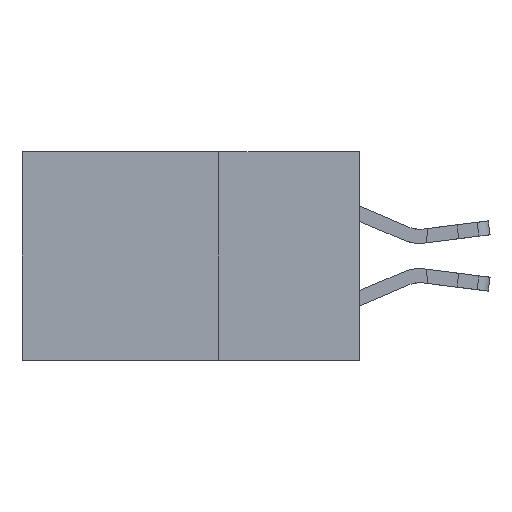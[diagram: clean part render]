
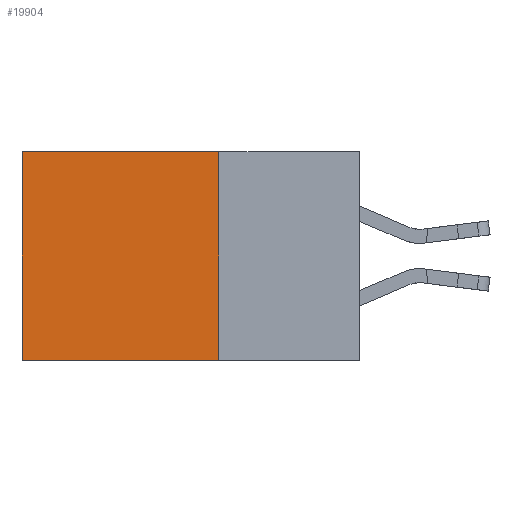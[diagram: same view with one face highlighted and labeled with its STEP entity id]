
A CAD part, left-side view. The second image highlights one B-rep face of the part: STEP entity #19904.
In plain terms, the highlighted planar face has unit normal (-1, 0, 0).
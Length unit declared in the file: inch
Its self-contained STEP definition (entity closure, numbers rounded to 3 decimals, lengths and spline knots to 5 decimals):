
#513 = EDGE_CURVE ( 'NONE', #1936, #17469, #19336, .T. ) ;
#823 = CARTESIAN_POINT ( 'NONE',  ( 0.2875, 0.25, 0. ) ) ;
#1936 = VERTEX_POINT ( 'NONE', #20392 ) ;
#2224 = CARTESIAN_POINT ( 'NONE',  ( 0.2875, 0.6, 0. ) ) ;
#2242 = EDGE_LOOP ( 'NONE', ( #12821, #14230, #16494, #14750 ) ) ;
#2592 = CARTESIAN_POINT ( 'NONE',  ( 0.2875, 0.25, 0. ) ) ;
#2720 = DIRECTION ( 'NONE',  ( 1., 0., 0. ) ) ;
#3605 = CARTESIAN_POINT ( 'NONE',  ( 0.2875, 0.25, -0.37 ) ) ;
#3711 = AXIS2_PLACEMENT_3D ( 'NONE', #823, #2720, #6047 ) ;
#5717 = DIRECTION ( 'NONE',  ( 0., 0., -1. ) ) ;
#6047 = DIRECTION ( 'NONE',  ( 0., 0., -1. ) ) ;
#6472 = VECTOR ( 'NONE', #8339, 39.37008 ) ;
#7638 = EDGE_CURVE ( 'NONE', #18789, #9838, #20378, .T. ) ;
#8339 = DIRECTION ( 'NONE',  ( 0., 1., 0. ) ) ;
#8608 = EDGE_CURVE ( 'NONE', #17469, #9838, #22026, .T. ) ;
#8977 = FACE_OUTER_BOUND ( 'NONE', #2242, .T. ) ;
#9171 = DIRECTION ( 'NONE',  ( 0., 1., 0. ) ) ;
#9616 = DIRECTION ( 'NONE',  ( 0., 0., -1. ) ) ;
#9838 = VERTEX_POINT ( 'NONE', #13046 ) ;
#12821 = ORIENTED_EDGE ( 'NONE', *, *, #7638, .T. ) ;
#13046 = CARTESIAN_POINT ( 'NONE',  ( 0.2875, 0.6, -0.37 ) ) ;
#14230 = ORIENTED_EDGE ( 'NONE', *, *, #8608, .F. ) ;
#14502 = VECTOR ( 'NONE', #9616, 39.37008 ) ;
#14750 = ORIENTED_EDGE ( 'NONE', *, *, #15107, .T. ) ;
#15107 = EDGE_CURVE ( 'NONE', #1936, #18789, #16398, .T. ) ;
#16398 = LINE ( 'NONE', #19269, #6472 ) ;
#16494 = ORIENTED_EDGE ( 'NONE', *, *, #513, .F. ) ;
#16640 = CARTESIAN_POINT ( 'NONE',  ( 0.2875, 0.25, -0.37 ) ) ;
#17469 = VERTEX_POINT ( 'NONE', #16640 ) ;
#18142 = PLANE ( 'NONE',  #3711 ) ;
#18789 = VERTEX_POINT ( 'NONE', #21118 ) ;
#18930 = VECTOR ( 'NONE', #9171, 39.37008 ) ;
#19269 = CARTESIAN_POINT ( 'NONE',  ( 0.2875, 0.25, 0. ) ) ;
#19336 = LINE ( 'NONE', #2592, #14502 ) ;
#19904 = ADVANCED_FACE ( 'NONE', ( #8977 ), #18142, .F. ) ;
#20107 = VECTOR ( 'NONE', #5717, 39.37008 ) ;
#20378 = LINE ( 'NONE', #2224, #20107 ) ;
#20392 = CARTESIAN_POINT ( 'NONE',  ( 0.2875, 0.25, 0. ) ) ;
#21118 = CARTESIAN_POINT ( 'NONE',  ( 0.2875, 0.6, 0. ) ) ;
#22026 = LINE ( 'NONE', #3605, #18930 ) ;
